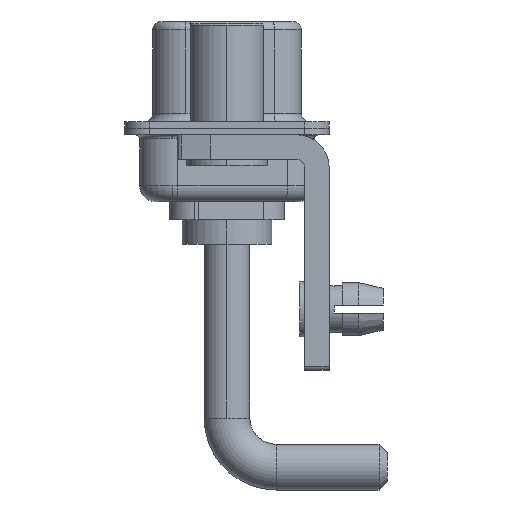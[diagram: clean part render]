
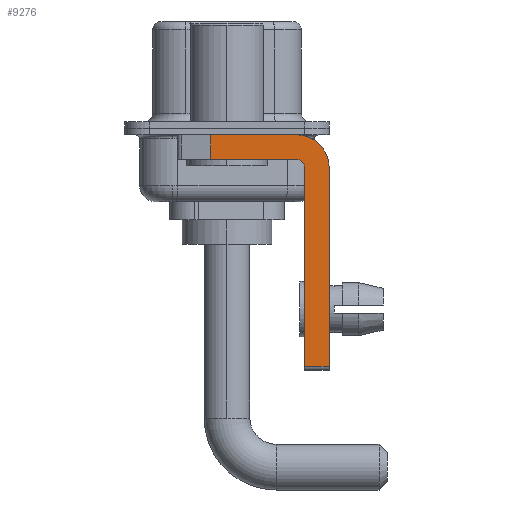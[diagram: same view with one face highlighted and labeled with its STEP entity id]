
A CAD part, left-side view. The second image highlights one B-rep face of the part: STEP entity #9276.
In plain terms, the highlighted planar face has unit normal (-1, 0, 0).
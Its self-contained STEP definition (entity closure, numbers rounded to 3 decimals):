
#172 = CIRCLE ( 'NONE', #12842, 2. ) ;
#515 = CARTESIAN_POINT ( 'NONE',  ( -2.9, -4.75, -14.55 ) ) ;
#714 = ORIENTED_EDGE ( 'NONE', *, *, #2403, .T. ) ;
#771 = EDGE_CURVE ( 'NONE', #8075, #1301, #172, .T. ) ;
#946 = EDGE_CURVE ( 'NONE', #1301, #2913, #5227, .T. ) ;
#1055 = CARTESIAN_POINT ( 'NONE',  ( -2.9, -4.75, -14.8 ) ) ;
#1154 = CARTESIAN_POINT ( 'NONE',  ( -2.9, -4.25, -2.4 ) ) ;
#1160 = ORIENTED_EDGE ( 'NONE', *, *, #946, .F. ) ;
#1301 = VERTEX_POINT ( 'NONE', #10370 ) ;
#1455 = DIRECTION ( 'NONE',  ( -1., 0., 0. ) ) ;
#1461 = VERTEX_POINT ( 'NONE', #515 ) ;
#2403 = EDGE_CURVE ( 'NONE', #1461, #2913, #11663, .T. ) ;
#2842 = VERTEX_POINT ( 'NONE', #11440 ) ;
#2913 = VERTEX_POINT ( 'NONE', #4510 ) ;
#3711 = EDGE_CURVE ( 'NONE', #14637, #8075, #9342, .T. ) ;
#4079 = CIRCLE ( 'NONE', #5671, 0.5 ) ;
#4476 = PLANE ( 'NONE',  #12119 ) ;
#4510 = CARTESIAN_POINT ( 'NONE',  ( -2.9, -6.25, -14.55 ) ) ;
#5227 = LINE ( 'NONE', #6327, #17922 ) ;
#5319 = EDGE_CURVE ( 'NONE', #1461, #2842, #16257, .T. ) ;
#5372 = EDGE_CURVE ( 'NONE', #2842, #16692, #4079, .T. ) ;
#5667 = CARTESIAN_POINT ( 'NONE',  ( -2.9, -4.25, -2.4 ) ) ;
#5671 = AXIS2_PLACEMENT_3D ( 'NONE', #1154, #1455, #10694 ) ;
#6327 = CARTESIAN_POINT ( 'NONE',  ( -2.9, -6.25, -2.4 ) ) ;
#6581 = LINE ( 'NONE', #16814, #14624 ) ;
#6740 = DIRECTION ( 'NONE',  ( 1., 0., 0. ) ) ;
#6934 = CARTESIAN_POINT ( 'NONE',  ( -2.9, -4.25, -2.4 ) ) ;
#7013 = VERTEX_POINT ( 'NONE', #10176 ) ;
#7629 = DIRECTION ( 'NONE',  ( 0., 0., -1. ) ) ;
#8075 = VERTEX_POINT ( 'NONE', #17515 ) ;
#8219 = ORIENTED_EDGE ( 'NONE', *, *, #18908, .T. ) ;
#8467 = EDGE_CURVE ( 'NONE', #16692, #7013, #6581, .T. ) ;
#8502 = CARTESIAN_POINT ( 'NONE',  ( -2.9, 0.978, -0.4 ) ) ;
#8857 = ORIENTED_EDGE ( 'NONE', *, *, #771, .F. ) ;
#9058 = ORIENTED_EDGE ( 'NONE', *, *, #8467, .F. ) ;
#9276 = ADVANCED_FACE ( 'NONE', ( #14886 ), #4476, .F. ) ;
#9342 = LINE ( 'NONE', #18735, #16426 ) ;
#10176 = CARTESIAN_POINT ( 'NONE',  ( -2.9, 0.978, -1.9 ) ) ;
#10370 = CARTESIAN_POINT ( 'NONE',  ( -2.9, -6.25, -2.4 ) ) ;
#10694 = DIRECTION ( 'NONE',  ( 0., 0., 1. ) ) ;
#10704 = ORIENTED_EDGE ( 'NONE', *, *, #5319, .F. ) ;
#10711 = VECTOR ( 'NONE', #15958, 1000. ) ;
#11440 = CARTESIAN_POINT ( 'NONE',  ( -2.9, -4.75, -2.4 ) ) ;
#11663 = LINE ( 'NONE', #14744, #18603 ) ;
#12119 = AXIS2_PLACEMENT_3D ( 'NONE', #5667, #14788, #16270 ) ;
#12475 = VECTOR ( 'NONE', #7629, 1000. ) ;
#12842 = AXIS2_PLACEMENT_3D ( 'NONE', #6934, #6740, #17257 ) ;
#13247 = DIRECTION ( 'NONE',  ( 0., -1., 0. ) ) ;
#14148 = DIRECTION ( 'NONE',  ( 0., 0., -1. ) ) ;
#14624 = VECTOR ( 'NONE', #15324, 1000. ) ;
#14637 = VERTEX_POINT ( 'NONE', #8502 ) ;
#14744 = CARTESIAN_POINT ( 'NONE',  ( -2.9, -4.25, -14.55 ) ) ;
#14788 = DIRECTION ( 'NONE',  ( 1., 0., 0. ) ) ;
#14886 = FACE_OUTER_BOUND ( 'NONE', #16587, .T. ) ;
#15324 = DIRECTION ( 'NONE',  ( 0., 1., 0. ) ) ;
#15684 = CARTESIAN_POINT ( 'NONE',  ( -2.9, -4.25, -1.9 ) ) ;
#15745 = ORIENTED_EDGE ( 'NONE', *, *, #5372, .F. ) ;
#15958 = DIRECTION ( 'NONE',  ( 0., 0., 1. ) ) ;
#16257 = LINE ( 'NONE', #1055, #10711 ) ;
#16270 = DIRECTION ( 'NONE',  ( 0., 0., -1. ) ) ;
#16426 = VECTOR ( 'NONE', #18549, 1000. ) ;
#16587 = EDGE_LOOP ( 'NONE', ( #18186, #8219, #9058, #15745, #10704, #714, #1160, #8857 ) ) ;
#16692 = VERTEX_POINT ( 'NONE', #15684 ) ;
#16814 = CARTESIAN_POINT ( 'NONE',  ( -2.9, -4.25, -1.9 ) ) ;
#17257 = DIRECTION ( 'NONE',  ( 0., 0., -1. ) ) ;
#17515 = CARTESIAN_POINT ( 'NONE',  ( -2.9, -4.25, -0.4 ) ) ;
#17922 = VECTOR ( 'NONE', #14148, 1000. ) ;
#18134 = CARTESIAN_POINT ( 'NONE',  ( -2.9, 0.978, -1.9 ) ) ;
#18186 = ORIENTED_EDGE ( 'NONE', *, *, #3711, .F. ) ;
#18422 = LINE ( 'NONE', #18134, #12475 ) ;
#18549 = DIRECTION ( 'NONE',  ( 0., -1., 0. ) ) ;
#18603 = VECTOR ( 'NONE', #13247, 1000. ) ;
#18735 = CARTESIAN_POINT ( 'NONE',  ( -2.9, 3., -0.4 ) ) ;
#18908 = EDGE_CURVE ( 'NONE', #14637, #7013, #18422, .T. ) ;
